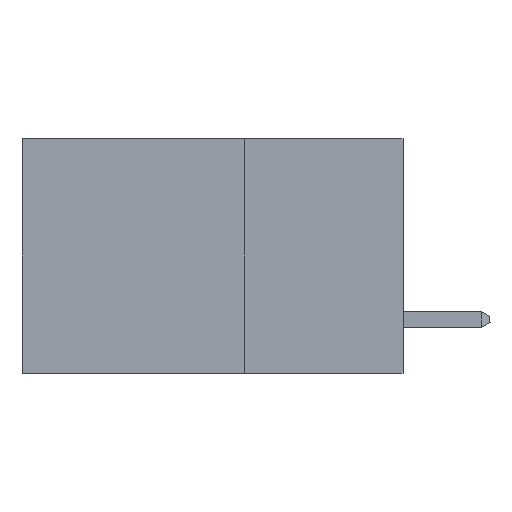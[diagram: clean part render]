
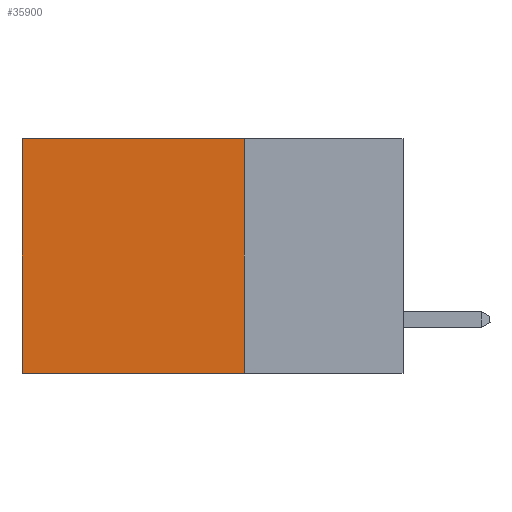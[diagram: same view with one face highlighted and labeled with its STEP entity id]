
A CAD part, left-side view. The second image highlights one B-rep face of the part: STEP entity #35900.
In plain terms, the highlighted planar face has unit normal (-1, 0, 0).
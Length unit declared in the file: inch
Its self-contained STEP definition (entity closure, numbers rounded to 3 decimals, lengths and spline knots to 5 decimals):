
#369 = VERTEX_POINT ( 'NONE', #9366 ) ;
#1734 = LINE ( 'NONE', #2900, #6329 ) ;
#2352 = CARTESIAN_POINT ( 'NONE',  ( 0.2875, 0.25, 0. ) ) ;
#2900 = CARTESIAN_POINT ( 'NONE',  ( 0.2875, 0.6, 0. ) ) ;
#5608 = CARTESIAN_POINT ( 'NONE',  ( 0.2875, 0.25, 0. ) ) ;
#5645 = LINE ( 'NONE', #8640, #10862 ) ;
#6134 = ORIENTED_EDGE ( 'NONE', *, *, #37187, .T. ) ;
#6329 = VECTOR ( 'NONE', #23441, 39.37008 ) ;
#8640 = CARTESIAN_POINT ( 'NONE',  ( 0.2875, 0.25, 0. ) ) ;
#8861 = VERTEX_POINT ( 'NONE', #5608 ) ;
#9334 = VERTEX_POINT ( 'NONE', #35532 ) ;
#9366 = CARTESIAN_POINT ( 'NONE',  ( 0.2875, 0.6, -0.37 ) ) ;
#9615 = EDGE_CURVE ( 'NONE', #9334, #369, #21798, .T. ) ;
#10862 = VECTOR ( 'NONE', #19073, 39.37008 ) ;
#11379 = EDGE_CURVE ( 'NONE', #38704, #369, #1734, .T. ) ;
#11543 = DIRECTION ( 'NONE',  ( 1., 0., 0. ) ) ;
#12970 = CARTESIAN_POINT ( 'NONE',  ( 0.2875, 0.6, 0. ) ) ;
#13106 = ORIENTED_EDGE ( 'NONE', *, *, #9615, .F. ) ;
#15660 = CARTESIAN_POINT ( 'NONE',  ( 0.2875, 0.25, -0.37 ) ) ;
#16618 = VECTOR ( 'NONE', #24949, 39.37008 ) ;
#17095 = EDGE_LOOP ( 'NONE', ( #21913, #13106, #23469, #6134 ) ) ;
#19073 = DIRECTION ( 'NONE',  ( 0., 0., -1. ) ) ;
#20643 = VECTOR ( 'NONE', #32271, 39.37008 ) ;
#21798 = LINE ( 'NONE', #15660, #16618 ) ;
#21913 = ORIENTED_EDGE ( 'NONE', *, *, #11379, .T. ) ;
#23441 = DIRECTION ( 'NONE',  ( 0., 0., -1. ) ) ;
#23469 = ORIENTED_EDGE ( 'NONE', *, *, #27203, .F. ) ;
#24949 = DIRECTION ( 'NONE',  ( 0., 1., 0. ) ) ;
#26806 = PLANE ( 'NONE',  #27692 ) ;
#27203 = EDGE_CURVE ( 'NONE', #8861, #9334, #5645, .T. ) ;
#27692 = AXIS2_PLACEMENT_3D ( 'NONE', #32488, #11543, #32633 ) ;
#31007 = LINE ( 'NONE', #2352, #20643 ) ;
#32271 = DIRECTION ( 'NONE',  ( 0., 1., 0. ) ) ;
#32488 = CARTESIAN_POINT ( 'NONE',  ( 0.2875, 0.25, 0. ) ) ;
#32633 = DIRECTION ( 'NONE',  ( 0., 0., -1. ) ) ;
#32953 = FACE_OUTER_BOUND ( 'NONE', #17095, .T. ) ;
#35532 = CARTESIAN_POINT ( 'NONE',  ( 0.2875, 0.25, -0.37 ) ) ;
#35900 = ADVANCED_FACE ( 'NONE', ( #32953 ), #26806, .F. ) ;
#37187 = EDGE_CURVE ( 'NONE', #8861, #38704, #31007, .T. ) ;
#38704 = VERTEX_POINT ( 'NONE', #12970 ) ;
